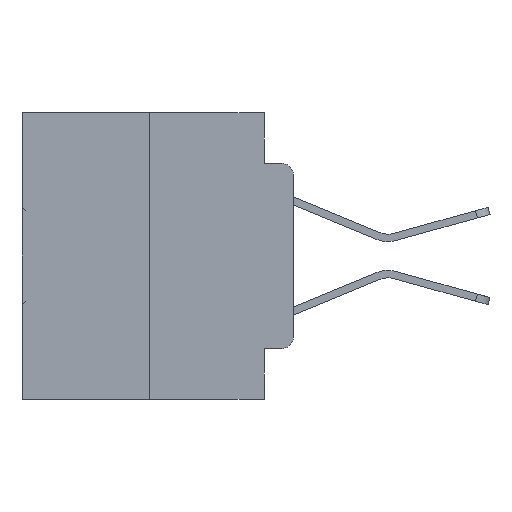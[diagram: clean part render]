
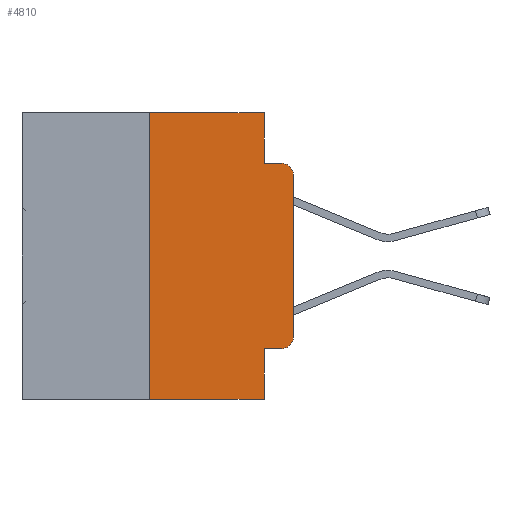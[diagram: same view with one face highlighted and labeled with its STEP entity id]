
A CAD part, left-side view. The second image highlights one B-rep face of the part: STEP entity #4810.
In plain terms, the highlighted planar face has unit normal (-1, 0, 0).
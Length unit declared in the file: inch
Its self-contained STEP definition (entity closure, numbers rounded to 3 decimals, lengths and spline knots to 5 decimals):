
#605 = LINE ( 'NONE', #2807, #21088 ) ;
#636 = LINE ( 'NONE', #1595, #26963 ) ;
#669 = ORIENTED_EDGE ( 'NONE', *, *, #27221, .F. ) ;
#1182 = DIRECTION ( 'NONE',  ( 0., 0., -1. ) ) ;
#1490 = VECTOR ( 'NONE', #14146, 39.37008 ) ;
#1595 = CARTESIAN_POINT ( 'NONE',  ( 0., 0., 0. ) ) ;
#2165 = LINE ( 'NONE', #31437, #21782 ) ;
#2462 = VERTEX_POINT ( 'NONE', #19154 ) ;
#2807 = CARTESIAN_POINT ( 'NONE',  ( 0., 0.051, -0.0885 ) ) ;
#3358 = CARTESIAN_POINT ( 'NONE',  ( 0., 0.051, -0.0885 ) ) ;
#3422 = DIRECTION ( 'NONE',  ( 0., 0., 1. ) ) ;
#4318 = VERTEX_POINT ( 'NONE', #29340 ) ;
#4767 = FACE_OUTER_BOUND ( 'NONE', #32079, .T. ) ;
#4810 = ADVANCED_FACE ( 'NONE', ( #4767 ), #8337, .F. ) ;
#4889 = EDGE_CURVE ( 'NONE', #13888, #16981, #21936, .T. ) ;
#5449 = LINE ( 'NONE', #14000, #11397 ) ;
#8043 = CARTESIAN_POINT ( 'NONE',  ( 0., 0.051, -0.4115 ) ) ;
#8337 = PLANE ( 'NONE',  #20485 ) ;
#8401 = CARTESIAN_POINT ( 'NONE',  ( 0., 0.473, 0. ) ) ;
#8479 = ORIENTED_EDGE ( 'NONE', *, *, #31458, .F. ) ;
#9160 = CIRCLE ( 'NONE', #32404, 0.02 ) ;
#9839 = VECTOR ( 'NONE', #30204, 39.37008 ) ;
#9944 = DIRECTION ( 'NONE',  ( 1., 0., 0. ) ) ;
#10013 = DIRECTION ( 'NONE',  ( 0., 0., -1. ) ) ;
#10236 = LINE ( 'NONE', #15081, #15495 ) ;
#10751 = CARTESIAN_POINT ( 'NONE',  ( 0., 0.02, -0.4115 ) ) ;
#11397 = VECTOR ( 'NONE', #1182, 39.37008 ) ;
#11580 = ORIENTED_EDGE ( 'NONE', *, *, #26668, .F. ) ;
#11821 = DIRECTION ( 'NONE',  ( -1., 0., 0. ) ) ;
#11905 = DIRECTION ( 'NONE',  ( 0., 0., 1. ) ) ;
#12152 = EDGE_CURVE ( 'NONE', #16981, #4318, #9160, .T. ) ;
#12542 = CARTESIAN_POINT ( 'NONE',  ( 0., 0.02, -0.1085 ) ) ;
#12679 = VERTEX_POINT ( 'NONE', #29164 ) ;
#13236 = VERTEX_POINT ( 'NONE', #18642 ) ;
#13512 = CARTESIAN_POINT ( 'NONE',  ( 0., 0.051, -0.4115 ) ) ;
#13628 = CARTESIAN_POINT ( 'NONE',  ( 0., 0.25, 0. ) ) ;
#13851 = DIRECTION ( 'NONE',  ( 0., -1., 0. ) ) ;
#13888 = VERTEX_POINT ( 'NONE', #8043 ) ;
#13986 = CIRCLE ( 'NONE', #17529, 0.02 ) ;
#14000 = CARTESIAN_POINT ( 'NONE',  ( 0., 0.051, 0. ) ) ;
#14146 = DIRECTION ( 'NONE',  ( 0., -1., 0. ) ) ;
#15058 = ORIENTED_EDGE ( 'NONE', *, *, #4889, .T. ) ;
#15081 = CARTESIAN_POINT ( 'NONE',  ( 0., 0.473, 0. ) ) ;
#15141 = DIRECTION ( 'NONE',  ( 0., 0., -1. ) ) ;
#15495 = VECTOR ( 'NONE', #30144, 39.37008 ) ;
#15866 = CARTESIAN_POINT ( 'NONE',  ( 0., 0.051, -0.5 ) ) ;
#16507 = VERTEX_POINT ( 'NONE', #29072 ) ;
#16706 = LINE ( 'NONE', #27711, #9839 ) ;
#16981 = VERTEX_POINT ( 'NONE', #10751 ) ;
#17529 = AXIS2_PLACEMENT_3D ( 'NONE', #12542, #30208, #15141 ) ;
#17838 = ORIENTED_EDGE ( 'NONE', *, *, #31206, .F. ) ;
#18151 = DIRECTION ( 'NONE',  ( 0., -1., 0. ) ) ;
#18642 = CARTESIAN_POINT ( 'NONE',  ( 0., 0.25, 0. ) ) ;
#19154 = CARTESIAN_POINT ( 'NONE',  ( 0., 0.051, 0. ) ) ;
#20485 = AXIS2_PLACEMENT_3D ( 'NONE', #8401, #9944, #10013 ) ;
#20802 = ORIENTED_EDGE ( 'NONE', *, *, #27274, .T. ) ;
#21088 = VECTOR ( 'NONE', #18151, 39.37008 ) ;
#21782 = VECTOR ( 'NONE', #13851, 39.37008 ) ;
#21936 = LINE ( 'NONE', #13512, #1490 ) ;
#22938 = EDGE_CURVE ( 'NONE', #2462, #26576, #16706, .T. ) ;
#23691 = VERTEX_POINT ( 'NONE', #25496 ) ;
#24816 = EDGE_CURVE ( 'NONE', #16507, #23691, #13986, .T. ) ;
#25496 = CARTESIAN_POINT ( 'NONE',  ( 0., 0.02, -0.0885 ) ) ;
#26576 = VERTEX_POINT ( 'NONE', #3358 ) ;
#26668 = EDGE_CURVE ( 'NONE', #13888, #32185, #5449, .T. ) ;
#26963 = VECTOR ( 'NONE', #11905, 39.37008 ) ;
#27047 = CARTESIAN_POINT ( 'NONE',  ( 0., 0.02, -0.3915 ) ) ;
#27221 = EDGE_CURVE ( 'NONE', #12679, #13236, #29985, .T. ) ;
#27274 = EDGE_CURVE ( 'NONE', #12679, #32185, #2165, .T. ) ;
#27711 = CARTESIAN_POINT ( 'NONE',  ( 0., 0.051, 0. ) ) ;
#27924 = ORIENTED_EDGE ( 'NONE', *, *, #24816, .T. ) ;
#28567 = ORIENTED_EDGE ( 'NONE', *, *, #12152, .T. ) ;
#28746 = ORIENTED_EDGE ( 'NONE', *, *, #22938, .F. ) ;
#29072 = CARTESIAN_POINT ( 'NONE',  ( 0., 0., -0.1085 ) ) ;
#29164 = CARTESIAN_POINT ( 'NONE',  ( 0., 0.25, -0.5 ) ) ;
#29200 = VECTOR ( 'NONE', #3422, 39.37008 ) ;
#29340 = CARTESIAN_POINT ( 'NONE',  ( 0., 0., -0.3915 ) ) ;
#29515 = DIRECTION ( 'NONE',  ( 0., 0., -1. ) ) ;
#29985 = LINE ( 'NONE', #13628, #29200 ) ;
#30048 = ORIENTED_EDGE ( 'NONE', *, *, #31025, .T. ) ;
#30144 = DIRECTION ( 'NONE',  ( 0., -1., 0. ) ) ;
#30204 = DIRECTION ( 'NONE',  ( 0., 0., -1. ) ) ;
#30208 = DIRECTION ( 'NONE',  ( -1., 0., 0. ) ) ;
#31025 = EDGE_CURVE ( 'NONE', #4318, #16507, #636, .T. ) ;
#31206 = EDGE_CURVE ( 'NONE', #13236, #2462, #10236, .T. ) ;
#31437 = CARTESIAN_POINT ( 'NONE',  ( 0., 0.473, -0.5 ) ) ;
#31458 = EDGE_CURVE ( 'NONE', #26576, #23691, #605, .T. ) ;
#32079 = EDGE_LOOP ( 'NONE', ( #30048, #27924, #8479, #28746, #17838, #669, #20802, #11580, #15058, #28567 ) ) ;
#32185 = VERTEX_POINT ( 'NONE', #15866 ) ;
#32404 = AXIS2_PLACEMENT_3D ( 'NONE', #27047, #11821, #29515 ) ;
